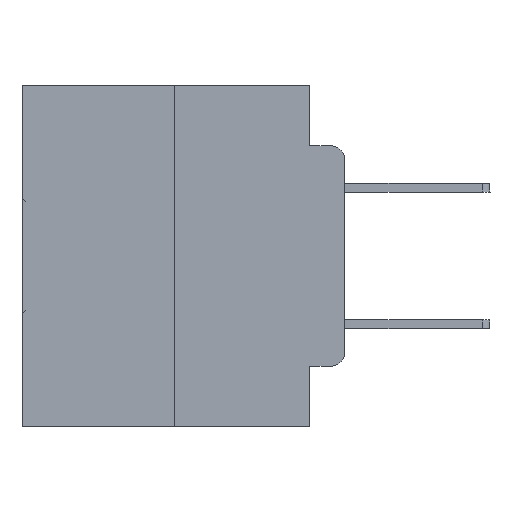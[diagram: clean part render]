
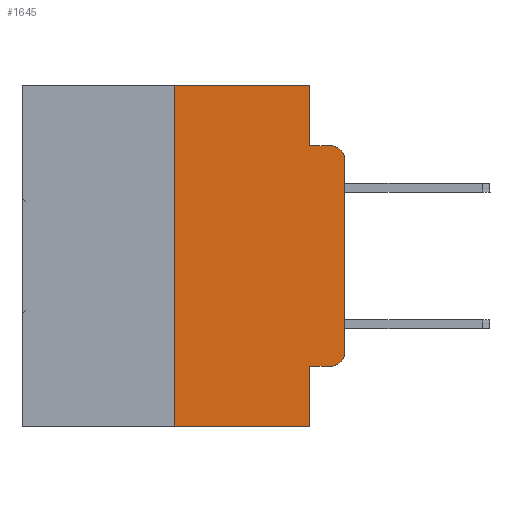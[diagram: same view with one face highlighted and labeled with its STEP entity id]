
A CAD part, left-side view. The second image highlights one B-rep face of the part: STEP entity #1645.
In plain terms, the highlighted planar face has unit normal (-1, 0, 0).
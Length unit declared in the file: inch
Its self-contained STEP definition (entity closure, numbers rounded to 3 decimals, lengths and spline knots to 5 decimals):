
#377 = ORIENTED_EDGE ( 'NONE', *, *, #13677, .F. ) ;
#387 = CARTESIAN_POINT ( 'NONE',  ( 0., 0.051, -0.0885 ) ) ;
#1011 = LINE ( 'NONE', #6007, #30320 ) ;
#1544 = VERTEX_POINT ( 'NONE', #20879 ) ;
#1645 = ADVANCED_FACE ( 'NONE', ( #29475 ), #9562, .F. ) ;
#2409 = CARTESIAN_POINT ( 'NONE',  ( 0., 0.02, -0.0885 ) ) ;
#2477 = CARTESIAN_POINT ( 'NONE',  ( 0., 0.473, 0. ) ) ;
#2827 = VECTOR ( 'NONE', #24832, 39.37008 ) ;
#3132 = ORIENTED_EDGE ( 'NONE', *, *, #8328, .T. ) ;
#3699 = CARTESIAN_POINT ( 'NONE',  ( 0., 0.25, -0.5 ) ) ;
#4387 = VERTEX_POINT ( 'NONE', #18261 ) ;
#4571 = EDGE_CURVE ( 'NONE', #26909, #9806, #5639, .T. ) ;
#5275 = CARTESIAN_POINT ( 'NONE',  ( 0., 0.051, 0. ) ) ;
#5639 = CIRCLE ( 'NONE', #28442, 0.02 ) ;
#6007 = CARTESIAN_POINT ( 'NONE',  ( 0., 0.25, 0. ) ) ;
#6045 = LINE ( 'NONE', #8178, #14027 ) ;
#6900 = CARTESIAN_POINT ( 'NONE',  ( 0., 0.051, 0. ) ) ;
#6902 = CARTESIAN_POINT ( 'NONE',  ( 0., 0.051, -0.4115 ) ) ;
#8178 = CARTESIAN_POINT ( 'NONE',  ( 0., 0.051, 0. ) ) ;
#8328 = EDGE_CURVE ( 'NONE', #25981, #4387, #12604, .T. ) ;
#8363 = EDGE_CURVE ( 'NONE', #28142, #29635, #29679, .T. ) ;
#9049 = VECTOR ( 'NONE', #30059, 39.37008 ) ;
#9085 = EDGE_CURVE ( 'NONE', #22834, #4387, #6045, .T. ) ;
#9190 = DIRECTION ( 'NONE',  ( 0., -1., 0. ) ) ;
#9295 = LINE ( 'NONE', #2477, #19711 ) ;
#9562 = PLANE ( 'NONE',  #25877 ) ;
#9662 = DIRECTION ( 'NONE',  ( 0., 0., -1. ) ) ;
#9806 = VERTEX_POINT ( 'NONE', #2409 ) ;
#9807 = LINE ( 'NONE', #387, #2827 ) ;
#10075 = VERTEX_POINT ( 'NONE', #30401 ) ;
#10610 = DIRECTION ( 'NONE',  ( 0., 0., -1. ) ) ;
#11240 = DIRECTION ( 'NONE',  ( -1., 0., 0. ) ) ;
#11408 = CARTESIAN_POINT ( 'NONE',  ( 0., 0.02, -0.1085 ) ) ;
#12604 = LINE ( 'NONE', #29935, #17196 ) ;
#13078 = DIRECTION ( 'NONE',  ( 0., -1., 0. ) ) ;
#13247 = EDGE_CURVE ( 'NONE', #29635, #26909, #25177, .T. ) ;
#13338 = ORIENTED_EDGE ( 'NONE', *, *, #25181, .F. ) ;
#13632 = AXIS2_PLACEMENT_3D ( 'NONE', #17605, #25530, #15494 ) ;
#13677 = EDGE_CURVE ( 'NONE', #10075, #9806, #9807, .T. ) ;
#13723 = LINE ( 'NONE', #6902, #24259 ) ;
#14027 = VECTOR ( 'NONE', #10610, 39.37008 ) ;
#14245 = CARTESIAN_POINT ( 'NONE',  ( 0., 0.473, 0. ) ) ;
#14411 = DIRECTION ( 'NONE',  ( 1., 0., 0. ) ) ;
#15494 = DIRECTION ( 'NONE',  ( 0., 0., -1. ) ) ;
#16406 = CARTESIAN_POINT ( 'NONE',  ( 0., 0.02, -0.4115 ) ) ;
#16565 = DIRECTION ( 'NONE',  ( 0., 0., -1. ) ) ;
#17196 = VECTOR ( 'NONE', #13078, 39.37008 ) ;
#17605 = CARTESIAN_POINT ( 'NONE',  ( 0., 0.02, -0.3915 ) ) ;
#17868 = ORIENTED_EDGE ( 'NONE', *, *, #21818, .F. ) ;
#18242 = ORIENTED_EDGE ( 'NONE', *, *, #8363, .T. ) ;
#18261 = CARTESIAN_POINT ( 'NONE',  ( 0., 0.051, -0.5 ) ) ;
#18439 = ORIENTED_EDGE ( 'NONE', *, *, #24529, .F. ) ;
#18879 = LINE ( 'NONE', #6900, #31293 ) ;
#19412 = CARTESIAN_POINT ( 'NONE',  ( 0., 0., -0.3915 ) ) ;
#19496 = VERTEX_POINT ( 'NONE', #5275 ) ;
#19701 = CARTESIAN_POINT ( 'NONE',  ( 0., 0.051, -0.4115 ) ) ;
#19711 = VECTOR ( 'NONE', #24319, 39.37008 ) ;
#20160 = CARTESIAN_POINT ( 'NONE',  ( 0., 0., 0. ) ) ;
#20628 = ORIENTED_EDGE ( 'NONE', *, *, #13247, .T. ) ;
#20879 = CARTESIAN_POINT ( 'NONE',  ( 0., 0.25, 0. ) ) ;
#21818 = EDGE_CURVE ( 'NONE', #1544, #19496, #9295, .T. ) ;
#22834 = VERTEX_POINT ( 'NONE', #19701 ) ;
#24259 = VECTOR ( 'NONE', #9190, 39.37008 ) ;
#24270 = DIRECTION ( 'NONE',  ( 0., 0., -1. ) ) ;
#24319 = DIRECTION ( 'NONE',  ( 0., -1., 0. ) ) ;
#24529 = EDGE_CURVE ( 'NONE', #19496, #10075, #18879, .T. ) ;
#24832 = DIRECTION ( 'NONE',  ( 0., -1., 0. ) ) ;
#25177 = LINE ( 'NONE', #20160, #9049 ) ;
#25181 = EDGE_CURVE ( 'NONE', #25981, #1544, #1011, .T. ) ;
#25446 = DIRECTION ( 'NONE',  ( 0., 0., 1. ) ) ;
#25530 = DIRECTION ( 'NONE',  ( -1., 0., 0. ) ) ;
#25877 = AXIS2_PLACEMENT_3D ( 'NONE', #14245, #14411, #24270 ) ;
#25981 = VERTEX_POINT ( 'NONE', #3699 ) ;
#26909 = VERTEX_POINT ( 'NONE', #29320 ) ;
#27113 = ORIENTED_EDGE ( 'NONE', *, *, #9085, .F. ) ;
#27820 = EDGE_LOOP ( 'NONE', ( #20628, #29681, #377, #18439, #17868, #13338, #3132, #27113, #29187, #18242 ) ) ;
#28142 = VERTEX_POINT ( 'NONE', #16406 ) ;
#28442 = AXIS2_PLACEMENT_3D ( 'NONE', #11408, #11240, #16565 ) ;
#28992 = EDGE_CURVE ( 'NONE', #22834, #28142, #13723, .T. ) ;
#29187 = ORIENTED_EDGE ( 'NONE', *, *, #28992, .T. ) ;
#29320 = CARTESIAN_POINT ( 'NONE',  ( 0., 0., -0.1085 ) ) ;
#29475 = FACE_OUTER_BOUND ( 'NONE', #27820, .T. ) ;
#29635 = VERTEX_POINT ( 'NONE', #19412 ) ;
#29679 = CIRCLE ( 'NONE', #13632, 0.02 ) ;
#29681 = ORIENTED_EDGE ( 'NONE', *, *, #4571, .T. ) ;
#29935 = CARTESIAN_POINT ( 'NONE',  ( 0., 0.473, -0.5 ) ) ;
#30059 = DIRECTION ( 'NONE',  ( 0., 0., 1. ) ) ;
#30320 = VECTOR ( 'NONE', #25446, 39.37008 ) ;
#30401 = CARTESIAN_POINT ( 'NONE',  ( 0., 0.051, -0.0885 ) ) ;
#31293 = VECTOR ( 'NONE', #9662, 39.37008 ) ;
